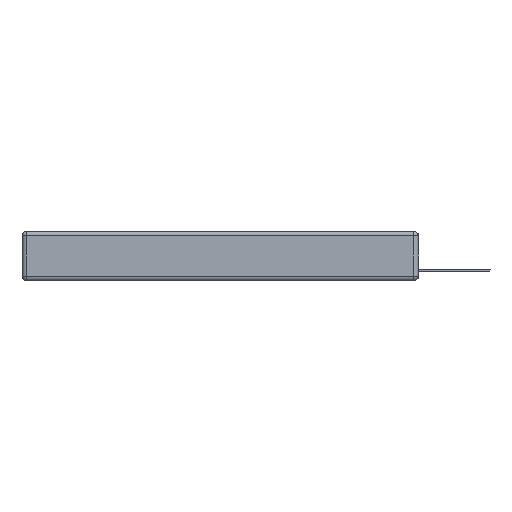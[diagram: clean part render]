
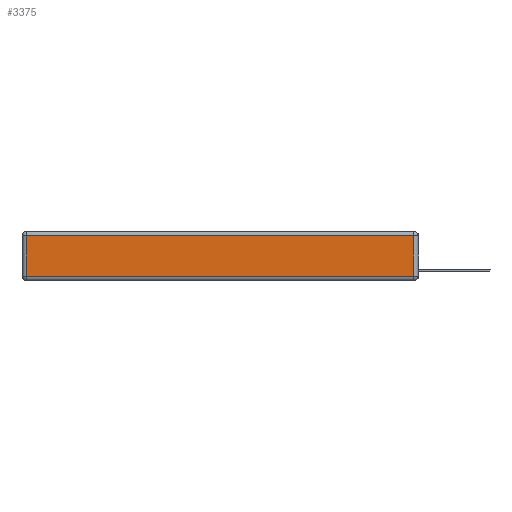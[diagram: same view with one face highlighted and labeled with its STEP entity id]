
A CAD part, left-side view. The second image highlights one B-rep face of the part: STEP entity #3375.
In plain terms, the highlighted planar face has unit normal (-1, 0, 0).
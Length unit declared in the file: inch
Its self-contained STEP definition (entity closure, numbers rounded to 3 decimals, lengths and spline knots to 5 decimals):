
#596 = DIRECTION ( 'NONE',  ( 0., 0., -1. ) ) ;
#918 = LINE ( 'NONE', #5633, #17562 ) ;
#1089 = EDGE_CURVE ( 'NONE', #8656, #9406, #16720, .T. ) ;
#2240 = DIRECTION ( 'NONE',  ( -1., 0., 0. ) ) ;
#2885 = ORIENTED_EDGE ( 'NONE', *, *, #3611, .T. ) ;
#3375 = ADVANCED_FACE ( 'NONE', ( #11964 ), #8860, .T. ) ;
#3611 = EDGE_CURVE ( 'NONE', #9406, #5655, #5497, .T. ) ;
#5048 = ORIENTED_EDGE ( 'NONE', *, *, #1089, .T. ) ;
#5497 = LINE ( 'NONE', #8390, #10725 ) ;
#5633 = CARTESIAN_POINT ( 'NONE',  ( 0., 2.72, -0.343 ) ) ;
#5655 = VERTEX_POINT ( 'NONE', #19675 ) ;
#6664 = VECTOR ( 'NONE', #19686, 39.37008 ) ;
#6733 = VERTEX_POINT ( 'NONE', #11231 ) ;
#6907 = AXIS2_PLACEMENT_3D ( 'NONE', #13993, #2240, #18384 ) ;
#7257 = VECTOR ( 'NONE', #19938, 39.37008 ) ;
#8390 = CARTESIAN_POINT ( 'NONE',  ( 0., 2.75, -0.03 ) ) ;
#8656 = VERTEX_POINT ( 'NONE', #9656 ) ;
#8860 = PLANE ( 'NONE',  #6907 ) ;
#9068 = LINE ( 'NONE', #20295, #6664 ) ;
#9406 = VERTEX_POINT ( 'NONE', #16116 ) ;
#9656 = CARTESIAN_POINT ( 'NONE',  ( 0., 0.03, -0.313 ) ) ;
#10194 = CARTESIAN_POINT ( 'NONE',  ( 0., 0.03, -0.343 ) ) ;
#10725 = VECTOR ( 'NONE', #13408, 39.37008 ) ;
#11231 = CARTESIAN_POINT ( 'NONE',  ( 0., 2.72, -0.313 ) ) ;
#11964 = FACE_OUTER_BOUND ( 'NONE', #12928, .T. ) ;
#12928 = EDGE_LOOP ( 'NONE', ( #18677, #5048, #2885, #13175 ) ) ;
#13175 = ORIENTED_EDGE ( 'NONE', *, *, #16097, .T. ) ;
#13408 = DIRECTION ( 'NONE',  ( 0., 1., 0. ) ) ;
#13993 = CARTESIAN_POINT ( 'NONE',  ( 0., 0., -0.343 ) ) ;
#16097 = EDGE_CURVE ( 'NONE', #5655, #6733, #918, .T. ) ;
#16116 = CARTESIAN_POINT ( 'NONE',  ( 0., 0.03, -0.03 ) ) ;
#16688 = EDGE_CURVE ( 'NONE', #6733, #8656, #9068, .T. ) ;
#16720 = LINE ( 'NONE', #10194, #7257 ) ;
#17562 = VECTOR ( 'NONE', #596, 39.37008 ) ;
#18384 = DIRECTION ( 'NONE',  ( 0., 0., 1. ) ) ;
#18677 = ORIENTED_EDGE ( 'NONE', *, *, #16688, .T. ) ;
#19675 = CARTESIAN_POINT ( 'NONE',  ( 0., 2.72, -0.03 ) ) ;
#19686 = DIRECTION ( 'NONE',  ( 0., -1., 0. ) ) ;
#19938 = DIRECTION ( 'NONE',  ( 0., 0., 1. ) ) ;
#20295 = CARTESIAN_POINT ( 'NONE',  ( 0., 0., -0.313 ) ) ;
